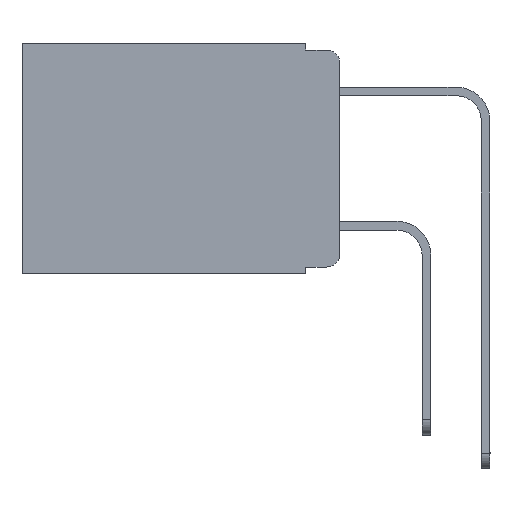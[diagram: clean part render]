
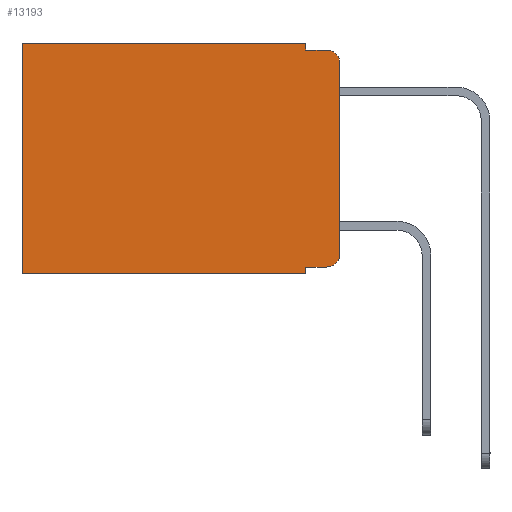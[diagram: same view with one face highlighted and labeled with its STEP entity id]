
A CAD part, left-side view. The second image highlights one B-rep face of the part: STEP entity #13193.
In plain terms, the highlighted planar face has unit normal (-1, 0, 0).
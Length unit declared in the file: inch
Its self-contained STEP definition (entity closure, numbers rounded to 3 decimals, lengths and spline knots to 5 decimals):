
#21 = VECTOR ( 'NONE', #4871, 39.37008 ) ;
#371 = DIRECTION ( 'NONE',  ( 0., 0., -1. ) ) ;
#711 = CARTESIAN_POINT ( 'NONE',  ( 0.298, 0.051, -0.333 ) ) ;
#833 = DIRECTION ( 'NONE',  ( 0., 1., 0. ) ) ;
#1336 = VERTEX_POINT ( 'NONE', #2941 ) ;
#1387 = CIRCLE ( 'NONE', #4553, 0.02 ) ;
#1536 = EDGE_CURVE ( 'NONE', #9837, #3724, #11649, .T. ) ;
#1652 = ORIENTED_EDGE ( 'NONE', *, *, #2354, .F. ) ;
#1664 = VECTOR ( 'NONE', #371, 39.37008 ) ;
#1751 = CARTESIAN_POINT ( 'NONE',  ( 0.298, 0.02, -0.333 ) ) ;
#1753 = CARTESIAN_POINT ( 'NONE',  ( 0.298, 0.473, 0. ) ) ;
#1755 = VERTEX_POINT ( 'NONE', #12042 ) ;
#2143 = CARTESIAN_POINT ( 'NONE',  ( 0.298, 0.02, -0.03 ) ) ;
#2354 = EDGE_CURVE ( 'NONE', #10629, #3060, #3949, .T. ) ;
#2600 = DIRECTION ( 'NONE',  ( 0., 0., -1. ) ) ;
#2697 = LINE ( 'NONE', #13421, #5273 ) ;
#2735 = CIRCLE ( 'NONE', #5446, 0.02 ) ;
#2778 = DIRECTION ( 'NONE',  ( 1., 0., 0. ) ) ;
#2812 = CARTESIAN_POINT ( 'NONE',  ( 0.298, 0.473, 0. ) ) ;
#2941 = CARTESIAN_POINT ( 'NONE',  ( 0.298, 0.051, 0. ) ) ;
#3009 = ORIENTED_EDGE ( 'NONE', *, *, #5272, .T. ) ;
#3060 = VERTEX_POINT ( 'NONE', #11130 ) ;
#3078 = CARTESIAN_POINT ( 'NONE',  ( 0.298, 0., -0.343 ) ) ;
#3306 = EDGE_LOOP ( 'NONE', ( #7224, #7820, #1652, #6734, #4032, #6998, #6546, #6720, #10008, #3009 ) ) ;
#3360 = CARTESIAN_POINT ( 'NONE',  ( 0.298, 0., -0.313 ) ) ;
#3443 = AXIS2_PLACEMENT_3D ( 'NONE', #5899, #2778, #11235 ) ;
#3635 = CARTESIAN_POINT ( 'NONE',  ( 0.298, 0.02, -0.313 ) ) ;
#3724 = VERTEX_POINT ( 'NONE', #1751 ) ;
#3831 = FACE_OUTER_BOUND ( 'NONE', #3306, .T. ) ;
#3944 = LINE ( 'NONE', #3078, #10262 ) ;
#3949 = LINE ( 'NONE', #7211, #6143 ) ;
#3950 = LINE ( 'NONE', #8347, #10479 ) ;
#4032 = ORIENTED_EDGE ( 'NONE', *, *, #12856, .T. ) ;
#4121 = CARTESIAN_POINT ( 'NONE',  ( 0.298, 0.473, -0.343 ) ) ;
#4194 = EDGE_CURVE ( 'NONE', #10724, #3060, #1387, .T. ) ;
#4553 = AXIS2_PLACEMENT_3D ( 'NONE', #2143, #13938, #12716 ) ;
#4664 = EDGE_CURVE ( 'NONE', #9837, #1755, #10898, .T. ) ;
#4690 = CARTESIAN_POINT ( 'NONE',  ( 0.298, 0.051, 0. ) ) ;
#4871 = DIRECTION ( 'NONE',  ( 0., 0., -1. ) ) ;
#4889 = VERTEX_POINT ( 'NONE', #1753 ) ;
#5272 = EDGE_CURVE ( 'NONE', #3724, #8113, #2735, .T. ) ;
#5273 = VECTOR ( 'NONE', #12284, 39.37008 ) ;
#5306 = DIRECTION ( 'NONE',  ( 0., 0., -1. ) ) ;
#5446 = AXIS2_PLACEMENT_3D ( 'NONE', #3635, #7988, #2600 ) ;
#5899 = CARTESIAN_POINT ( 'NONE',  ( 0.298, 0., 0. ) ) ;
#6143 = VECTOR ( 'NONE', #9265, 39.37008 ) ;
#6275 = CARTESIAN_POINT ( 'NONE',  ( 0.298, 0.051, -0.333 ) ) ;
#6546 = ORIENTED_EDGE ( 'NONE', *, *, #9851, .F. ) ;
#6720 = ORIENTED_EDGE ( 'NONE', *, *, #4664, .F. ) ;
#6734 = ORIENTED_EDGE ( 'NONE', *, *, #10484, .F. ) ;
#6998 = ORIENTED_EDGE ( 'NONE', *, *, #7017, .T. ) ;
#7017 = EDGE_CURVE ( 'NONE', #4889, #10209, #8200, .T. ) ;
#7106 = CARTESIAN_POINT ( 'NONE',  ( 0.298, 0.051, -0.01 ) ) ;
#7211 = CARTESIAN_POINT ( 'NONE',  ( 0.298, 0.051, -0.01 ) ) ;
#7224 = ORIENTED_EDGE ( 'NONE', *, *, #9108, .F. ) ;
#7820 = ORIENTED_EDGE ( 'NONE', *, *, #4194, .T. ) ;
#7988 = DIRECTION ( 'NONE',  ( -1., 0., 0. ) ) ;
#8113 = VERTEX_POINT ( 'NONE', #3360 ) ;
#8173 = PLANE ( 'NONE',  #3443 ) ;
#8200 = LINE ( 'NONE', #2812, #21 ) ;
#8347 = CARTESIAN_POINT ( 'NONE',  ( 0.298, 0., 0. ) ) ;
#9108 = EDGE_CURVE ( 'NONE', #10724, #8113, #2697, .T. ) ;
#9265 = DIRECTION ( 'NONE',  ( 0., -1., 0. ) ) ;
#9837 = VERTEX_POINT ( 'NONE', #6275 ) ;
#9851 = EDGE_CURVE ( 'NONE', #1755, #10209, #3944, .T. ) ;
#9938 = VECTOR ( 'NONE', #12633, 39.37008 ) ;
#9941 = LINE ( 'NONE', #4690, #1664 ) ;
#10008 = ORIENTED_EDGE ( 'NONE', *, *, #1536, .T. ) ;
#10209 = VERTEX_POINT ( 'NONE', #4121 ) ;
#10262 = VECTOR ( 'NONE', #13871, 39.37008 ) ;
#10479 = VECTOR ( 'NONE', #833, 39.37008 ) ;
#10484 = EDGE_CURVE ( 'NONE', #1336, #10629, #9941, .T. ) ;
#10629 = VERTEX_POINT ( 'NONE', #7106 ) ;
#10695 = CARTESIAN_POINT ( 'NONE',  ( 0.298, 0.051, 0. ) ) ;
#10724 = VERTEX_POINT ( 'NONE', #11438 ) ;
#10898 = LINE ( 'NONE', #10695, #13407 ) ;
#11130 = CARTESIAN_POINT ( 'NONE',  ( 0.298, 0.02, -0.01 ) ) ;
#11235 = DIRECTION ( 'NONE',  ( 0., 0., -1. ) ) ;
#11438 = CARTESIAN_POINT ( 'NONE',  ( 0.298, 0., -0.03 ) ) ;
#11649 = LINE ( 'NONE', #711, #9938 ) ;
#12042 = CARTESIAN_POINT ( 'NONE',  ( 0.298, 0.051, -0.343 ) ) ;
#12284 = DIRECTION ( 'NONE',  ( 0., 0., -1. ) ) ;
#12633 = DIRECTION ( 'NONE',  ( 0., -1., 0. ) ) ;
#12716 = DIRECTION ( 'NONE',  ( 0., 0., -1. ) ) ;
#12856 = EDGE_CURVE ( 'NONE', #1336, #4889, #3950, .T. ) ;
#13193 = ADVANCED_FACE ( 'NONE', ( #3831 ), #8173, .F. ) ;
#13407 = VECTOR ( 'NONE', #5306, 39.37008 ) ;
#13421 = CARTESIAN_POINT ( 'NONE',  ( 0.298, 0., 0. ) ) ;
#13871 = DIRECTION ( 'NONE',  ( 0., 1., 0. ) ) ;
#13938 = DIRECTION ( 'NONE',  ( -1., 0., 0. ) ) ;
